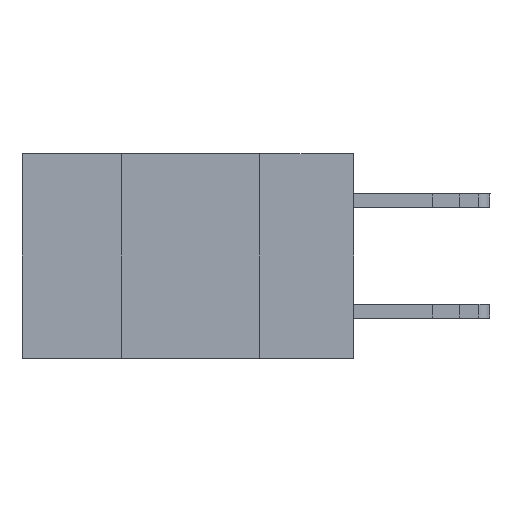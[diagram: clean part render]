
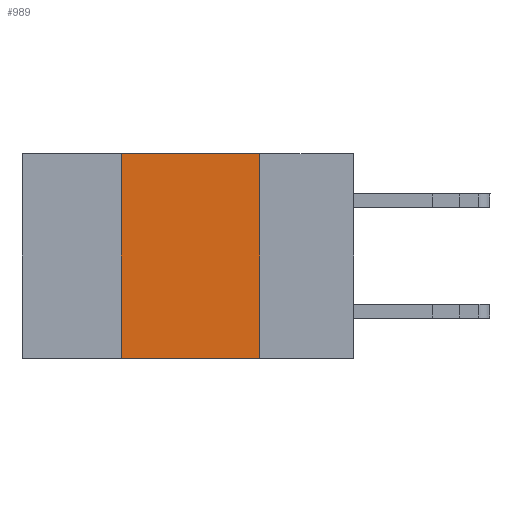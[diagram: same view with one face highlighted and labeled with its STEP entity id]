
A CAD part, left-side view. The second image highlights one B-rep face of the part: STEP entity #989.
In plain terms, the highlighted planar face has unit normal (-1, 0, 0).
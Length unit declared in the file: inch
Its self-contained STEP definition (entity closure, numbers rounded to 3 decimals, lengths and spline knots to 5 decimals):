
#387 = VERTEX_POINT ( 'NONE', #9437 ) ;
#425 = FACE_OUTER_BOUND ( 'NONE', #21676, .T. ) ;
#441 = AXIS2_PLACEMENT_3D ( 'NONE', #12821, #18764, #5434 ) ;
#989 = ADVANCED_FACE ( 'NONE', ( #425 ), #12918, .F. ) ;
#1628 = LINE ( 'NONE', #4776, #11991 ) ;
#3123 = ORIENTED_EDGE ( 'NONE', *, *, #20571, .F. ) ;
#3324 = VERTEX_POINT ( 'NONE', #10910 ) ;
#3439 = ORIENTED_EDGE ( 'NONE', *, *, #14049, .F. ) ;
#4776 = CARTESIAN_POINT ( 'NONE',  ( 0., 0.42, 0. ) ) ;
#4979 = DIRECTION ( 'NONE',  ( 0., 0., -1. ) ) ;
#5434 = DIRECTION ( 'NONE',  ( 0., 0., -1. ) ) ;
#6383 = CARTESIAN_POINT ( 'NONE',  ( 0., 0.17, 0. ) ) ;
#6805 = LINE ( 'NONE', #6383, #20141 ) ;
#7424 = CARTESIAN_POINT ( 'NONE',  ( 0., 0.42, 0. ) ) ;
#7498 = VECTOR ( 'NONE', #7652, 39.37008 ) ;
#7652 = DIRECTION ( 'NONE',  ( 0., -1., 0. ) ) ;
#7979 = DIRECTION ( 'NONE',  ( 0., 0., 1. ) ) ;
#8537 = EDGE_CURVE ( 'NONE', #15854, #3324, #14577, .T. ) ;
#9437 = CARTESIAN_POINT ( 'NONE',  ( 0., 0.17, 0. ) ) ;
#10850 = CARTESIAN_POINT ( 'NONE',  ( 0., 0.6, -0.37 ) ) ;
#10910 = CARTESIAN_POINT ( 'NONE',  ( 0., 0.17, -0.37 ) ) ;
#11991 = VECTOR ( 'NONE', #7979, 39.37008 ) ;
#12534 = LINE ( 'NONE', #17294, #13988 ) ;
#12821 = CARTESIAN_POINT ( 'NONE',  ( 0., 0.6, 0. ) ) ;
#12918 = PLANE ( 'NONE',  #441 ) ;
#13904 = CARTESIAN_POINT ( 'NONE',  ( 0., 0.42, -0.37 ) ) ;
#13988 = VECTOR ( 'NONE', #22705, 39.37008 ) ;
#14049 = EDGE_CURVE ( 'NONE', #20856, #387, #12534, .T. ) ;
#14577 = LINE ( 'NONE', #10850, #7498 ) ;
#15854 = VERTEX_POINT ( 'NONE', #13904 ) ;
#17241 = EDGE_CURVE ( 'NONE', #387, #3324, #6805, .T. ) ;
#17294 = CARTESIAN_POINT ( 'NONE',  ( 0., 0.6, 0. ) ) ;
#18764 = DIRECTION ( 'NONE',  ( 1., 0., 0. ) ) ;
#20141 = VECTOR ( 'NONE', #4979, 39.37008 ) ;
#20571 = EDGE_CURVE ( 'NONE', #15854, #20856, #1628, .T. ) ;
#20856 = VERTEX_POINT ( 'NONE', #7424 ) ;
#21676 = EDGE_LOOP ( 'NONE', ( #22282, #3439, #3123, #22060 ) ) ;
#22060 = ORIENTED_EDGE ( 'NONE', *, *, #8537, .T. ) ;
#22282 = ORIENTED_EDGE ( 'NONE', *, *, #17241, .F. ) ;
#22705 = DIRECTION ( 'NONE',  ( 0., -1., 0. ) ) ;
